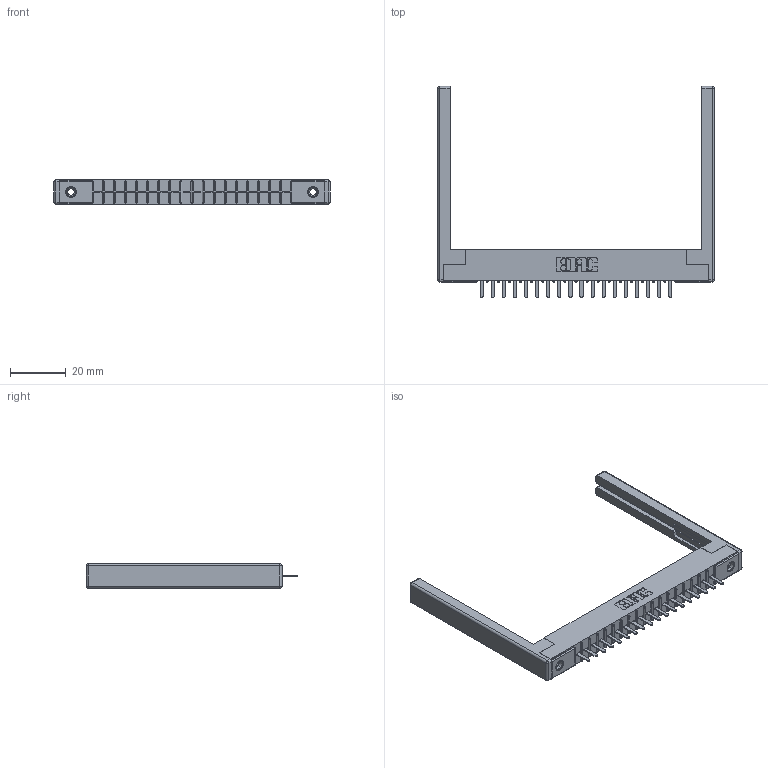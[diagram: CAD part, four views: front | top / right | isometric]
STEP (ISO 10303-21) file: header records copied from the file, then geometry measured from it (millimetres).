
FILE_DESCRIPTION (( 'STEP AP203' ), '1' );
FILE_NAME ('316-018-420-168.STEP', '2020-09-22T18:43:14', ( '' ), ( '' ), 'SwSTEP 2.0', 'SolidWorks 2020', '' );
FILE_SCHEMA (( 'CONFIG_CONTROL_DESIGN' ));
Length unit declared in the file: inch
Products named in the file (5): 306-290-001_120; 306 Part_.156 Dia; 345-250-001_345-250-001-102; 316-018-420-168; 307-220-068
Assembly tree (23 placements, depth 2):
  316-018-420-168
    306 Part_.156 Dia
    306-290-001_120  x18
    345-250-001_345-250-001-102  x2
    307-220-068  x2
Bounding box: 98.76 x 75.41 x 8.71 mm (x, y, z)
Volume: 11291.3 mm3; surface area: 13948.9 mm2
Topology: 23 solids, 23 shells, 1530 faces, 4252 edges, 2716 vertices
Faces by surface type: plane 1002, cylinder 432, sphere 80, cone 12, torus 4
Entity records: 22610 total; most frequent: CARTESIAN_POINT 3758, DIRECTION 3721, ORIENTED_EDGE 3714, EDGE_CURVE 1857, VECTOR 1435, LINE 1435, VERTEX_POINT 1180, AXIS2_PLACEMENT_3D 1143
